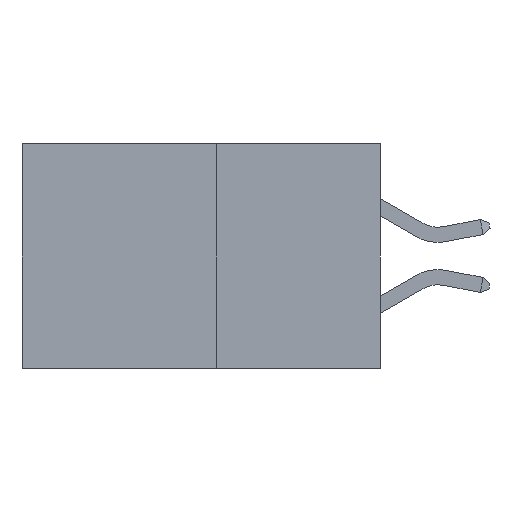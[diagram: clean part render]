
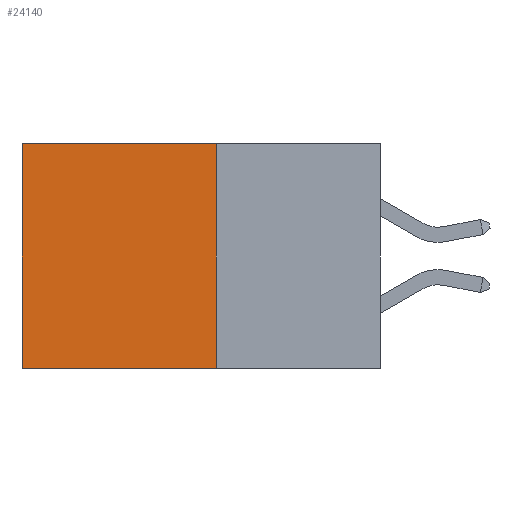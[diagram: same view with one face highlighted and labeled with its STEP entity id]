
A CAD part, left-side view. The second image highlights one B-rep face of the part: STEP entity #24140.
In plain terms, the highlighted planar face has unit normal (-1, 0, 0).
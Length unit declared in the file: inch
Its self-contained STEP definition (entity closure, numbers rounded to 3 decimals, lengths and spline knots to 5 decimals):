
#901 = VECTOR ( 'NONE', #12385, 39.37008 ) ;
#1674 = VECTOR ( 'NONE', #4502, 39.37008 ) ;
#2315 = DIRECTION ( 'NONE',  ( 0., 0., -1. ) ) ;
#2478 = ORIENTED_EDGE ( 'NONE', *, *, #13983, .F. ) ;
#3428 = EDGE_CURVE ( 'NONE', #18256, #6490, #19124, .T. ) ;
#3623 = VERTEX_POINT ( 'NONE', #12730 ) ;
#4502 = DIRECTION ( 'NONE',  ( 0., 1., 0. ) ) ;
#5539 = FACE_OUTER_BOUND ( 'NONE', #28290, .T. ) ;
#6090 = LINE ( 'NONE', #7104, #18872 ) ;
#6490 = VERTEX_POINT ( 'NONE', #26962 ) ;
#7104 = CARTESIAN_POINT ( 'NONE',  ( 0.277, 0.27, -0.37 ) ) ;
#7843 = LINE ( 'NONE', #9218, #19185 ) ;
#8378 = DIRECTION ( 'NONE',  ( 1., 0., 0. ) ) ;
#9218 = CARTESIAN_POINT ( 'NONE',  ( 0.277, 0.59, -0.37 ) ) ;
#9282 = ORIENTED_EDGE ( 'NONE', *, *, #20102, .F. ) ;
#9624 = ORIENTED_EDGE ( 'NONE', *, *, #3428, .T. ) ;
#9977 = EDGE_CURVE ( 'NONE', #6490, #13166, #7843, .T. ) ;
#12385 = DIRECTION ( 'NONE',  ( 0., 0., -1. ) ) ;
#12730 = CARTESIAN_POINT ( 'NONE',  ( 0.277, 0.27, -0.37 ) ) ;
#13032 = LINE ( 'NONE', #23649, #901 ) ;
#13166 = VERTEX_POINT ( 'NONE', #13695 ) ;
#13695 = CARTESIAN_POINT ( 'NONE',  ( 0.277, 0.59, -0.37 ) ) ;
#13983 = EDGE_CURVE ( 'NONE', #18256, #3623, #13032, .T. ) ;
#15302 = ORIENTED_EDGE ( 'NONE', *, *, #9977, .T. ) ;
#15773 = CARTESIAN_POINT ( 'NONE',  ( 0.277, 0.27, 0. ) ) ;
#15826 = CARTESIAN_POINT ( 'NONE',  ( 0.277, 0.27, 0. ) ) ;
#18256 = VERTEX_POINT ( 'NONE', #15773 ) ;
#18872 = VECTOR ( 'NONE', #22853, 39.37008 ) ;
#19124 = LINE ( 'NONE', #15826, #1674 ) ;
#19185 = VECTOR ( 'NONE', #2315, 39.37008 ) ;
#19651 = PLANE ( 'NONE',  #20585 ) ;
#20102 = EDGE_CURVE ( 'NONE', #3623, #13166, #6090, .T. ) ;
#20585 = AXIS2_PLACEMENT_3D ( 'NONE', #26282, #8378, #24165 ) ;
#22853 = DIRECTION ( 'NONE',  ( 0., 1., 0. ) ) ;
#23649 = CARTESIAN_POINT ( 'NONE',  ( 0.277, 0.27, -0.37 ) ) ;
#24140 = ADVANCED_FACE ( 'NONE', ( #5539 ), #19651, .F. ) ;
#24165 = DIRECTION ( 'NONE',  ( 0., 0., -1. ) ) ;
#26282 = CARTESIAN_POINT ( 'NONE',  ( 0.277, 0.27, -0.37 ) ) ;
#26962 = CARTESIAN_POINT ( 'NONE',  ( 0.277, 0.59, 0. ) ) ;
#28290 = EDGE_LOOP ( 'NONE', ( #15302, #9282, #2478, #9624 ) ) ;
